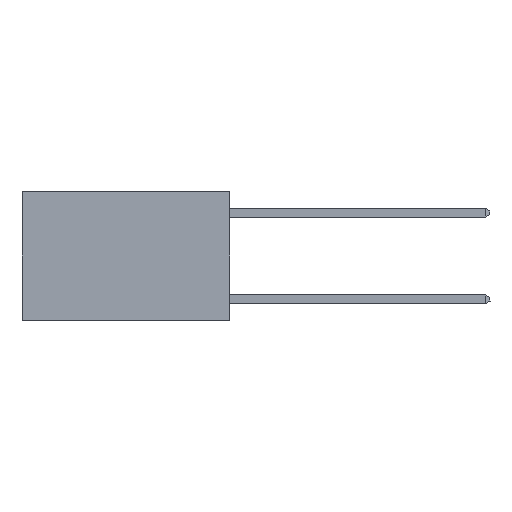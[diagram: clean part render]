
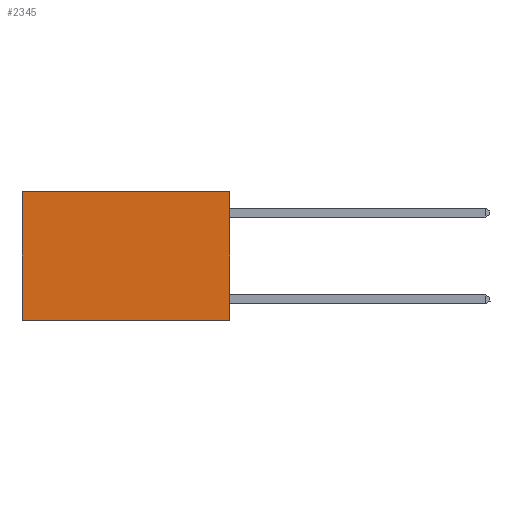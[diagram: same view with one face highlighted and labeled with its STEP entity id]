
A CAD part, left-side view. The second image highlights one B-rep face of the part: STEP entity #2345.
In plain terms, the highlighted planar face has unit normal (-1, 0, 0).
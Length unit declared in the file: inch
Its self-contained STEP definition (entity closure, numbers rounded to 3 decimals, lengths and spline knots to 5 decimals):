
#314 = LINE ( 'NONE', #1887, #10655 ) ;
#448 = VERTEX_POINT ( 'NONE', #7677 ) ;
#783 = DIRECTION ( 'NONE',  ( 0., 0., -1. ) ) ;
#822 = DIRECTION ( 'NONE',  ( 0., 1., 0. ) ) ;
#1363 = VECTOR ( 'NONE', #9825, 39.37008 ) ;
#1426 = LINE ( 'NONE', #7435, #4060 ) ;
#1887 = CARTESIAN_POINT ( 'NONE',  ( 0.2625, 0., 0. ) ) ;
#2345 = ADVANCED_FACE ( 'NONE', ( #5810 ), #5157, .F. ) ;
#2807 = VERTEX_POINT ( 'NONE', #12713 ) ;
#2920 = ORIENTED_EDGE ( 'NONE', *, *, #9485, .F. ) ;
#3126 = EDGE_LOOP ( 'NONE', ( #7530, #12888, #2920, #5767 ) ) ;
#3894 = AXIS2_PLACEMENT_3D ( 'NONE', #6189, #7246, #783 ) ;
#3931 = EDGE_CURVE ( 'NONE', #10126, #2807, #6097, .T. ) ;
#3940 = EDGE_CURVE ( 'NONE', #448, #8614, #314, .T. ) ;
#4060 = VECTOR ( 'NONE', #8388, 39.37008 ) ;
#4899 = CARTESIAN_POINT ( 'NONE',  ( 0.2625, 0., 0. ) ) ;
#5157 = PLANE ( 'NONE',  #3894 ) ;
#5767 = ORIENTED_EDGE ( 'NONE', *, *, #3940, .T. ) ;
#5775 = VECTOR ( 'NONE', #12000, 39.37008 ) ;
#5810 = FACE_OUTER_BOUND ( 'NONE', #3126, .T. ) ;
#6097 = LINE ( 'NONE', #11067, #5775 ) ;
#6189 = CARTESIAN_POINT ( 'NONE',  ( 0.2625, 0., 0. ) ) ;
#6584 = EDGE_CURVE ( 'NONE', #8614, #2807, #1426, .T. ) ;
#6875 = CARTESIAN_POINT ( 'NONE',  ( 0.2625, 0., -0.37 ) ) ;
#7246 = DIRECTION ( 'NONE',  ( 1., 0., 0. ) ) ;
#7435 = CARTESIAN_POINT ( 'NONE',  ( 0.2625, 0.6, 0. ) ) ;
#7530 = ORIENTED_EDGE ( 'NONE', *, *, #6584, .T. ) ;
#7677 = CARTESIAN_POINT ( 'NONE',  ( 0.2625, 0., 0. ) ) ;
#8388 = DIRECTION ( 'NONE',  ( 0., 0., -1. ) ) ;
#8614 = VERTEX_POINT ( 'NONE', #12617 ) ;
#9485 = EDGE_CURVE ( 'NONE', #448, #10126, #11869, .T. ) ;
#9825 = DIRECTION ( 'NONE',  ( 0., 0., -1. ) ) ;
#10126 = VERTEX_POINT ( 'NONE', #6875 ) ;
#10655 = VECTOR ( 'NONE', #822, 39.37008 ) ;
#11067 = CARTESIAN_POINT ( 'NONE',  ( 0.2625, 0., -0.37 ) ) ;
#11869 = LINE ( 'NONE', #4899, #1363 ) ;
#12000 = DIRECTION ( 'NONE',  ( 0., 1., 0. ) ) ;
#12617 = CARTESIAN_POINT ( 'NONE',  ( 0.2625, 0.6, 0. ) ) ;
#12713 = CARTESIAN_POINT ( 'NONE',  ( 0.2625, 0.6, -0.37 ) ) ;
#12888 = ORIENTED_EDGE ( 'NONE', *, *, #3931, .F. ) ;
